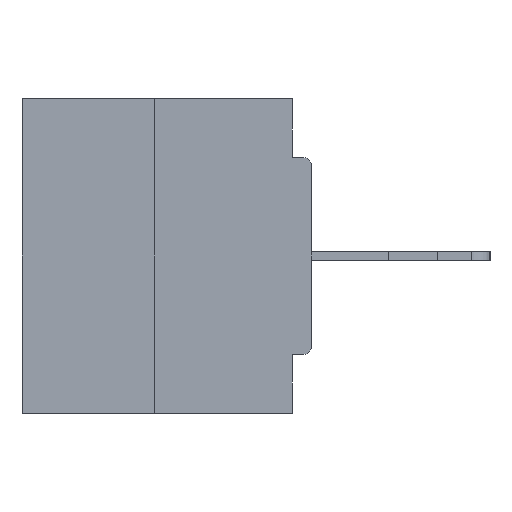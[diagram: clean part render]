
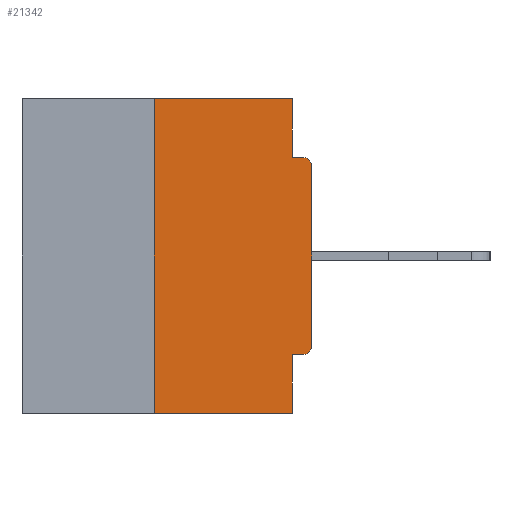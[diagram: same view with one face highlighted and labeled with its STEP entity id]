
A CAD part, left-side view. The second image highlights one B-rep face of the part: STEP entity #21342.
In plain terms, the highlighted planar face has unit normal (-1, 0, 0).
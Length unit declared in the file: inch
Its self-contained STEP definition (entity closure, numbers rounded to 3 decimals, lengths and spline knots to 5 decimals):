
#520 = DIRECTION ( 'NONE',  ( 1., 0., 0. ) ) ;
#844 = DIRECTION ( 'NONE',  ( 0., -1., 0. ) ) ;
#1271 = CARTESIAN_POINT ( 'NONE',  ( 0., 0.031, 0. ) ) ;
#1553 = VERTEX_POINT ( 'NONE', #24819 ) ;
#1582 = VERTEX_POINT ( 'NONE', #28336 ) ;
#1610 = VECTOR ( 'NONE', #22622, 39.37008 ) ;
#2001 = CIRCLE ( 'NONE', #3711, 0.015 ) ;
#2965 = VERTEX_POINT ( 'NONE', #4468 ) ;
#3505 = VECTOR ( 'NONE', #28901, 39.37008 ) ;
#3711 = AXIS2_PLACEMENT_3D ( 'NONE', #12974, #24083, #13518 ) ;
#3840 = VECTOR ( 'NONE', #9490, 39.37008 ) ;
#3979 = EDGE_CURVE ( 'NONE', #10822, #13764, #24867, .T. ) ;
#4160 = VECTOR ( 'NONE', #13693, 39.37008 ) ;
#4359 = CARTESIAN_POINT ( 'NONE',  ( 0., 0.015, -0.4065 ) ) ;
#4405 = DIRECTION ( 'NONE',  ( 0., 0., -1. ) ) ;
#4468 = CARTESIAN_POINT ( 'NONE',  ( 0., 0.25, -0.5 ) ) ;
#5059 = DIRECTION ( 'NONE',  ( 0., 0., 1. ) ) ;
#5913 = ORIENTED_EDGE ( 'NONE', *, *, #20773, .T. ) ;
#6026 = CARTESIAN_POINT ( 'NONE',  ( 0., 0., -0.3915 ) ) ;
#6584 = EDGE_LOOP ( 'NONE', ( #23778, #14687, #17450, #22697, #16497, #25538, #15675, #5913, #7654, #16845 ) ) ;
#7648 = EDGE_CURVE ( 'NONE', #10822, #25577, #26521, .T. ) ;
#7654 = ORIENTED_EDGE ( 'NONE', *, *, #25729, .F. ) ;
#8344 = CARTESIAN_POINT ( 'NONE',  ( 0., 0.031, -0.5 ) ) ;
#8827 = CARTESIAN_POINT ( 'NONE',  ( 0., 0., -0.0935 ) ) ;
#8965 = CARTESIAN_POINT ( 'NONE',  ( 0., 0.25, 0. ) ) ;
#9369 = DIRECTION ( 'NONE',  ( -1., 0., 0. ) ) ;
#9383 = VECTOR ( 'NONE', #10090, 39.37008 ) ;
#9490 = DIRECTION ( 'NONE',  ( 0., -1., 0. ) ) ;
#9552 = VERTEX_POINT ( 'NONE', #8965 ) ;
#9813 = CARTESIAN_POINT ( 'NONE',  ( 0., 0., 0. ) ) ;
#10090 = DIRECTION ( 'NONE',  ( 0., 1., 0. ) ) ;
#10709 = EDGE_CURVE ( 'NONE', #9552, #1582, #19611, .T. ) ;
#10822 = VERTEX_POINT ( 'NONE', #4359 ) ;
#11756 = VECTOR ( 'NONE', #5059, 39.37008 ) ;
#11995 = CARTESIAN_POINT ( 'NONE',  ( 0., 0.46, -0.5 ) ) ;
#12761 = CARTESIAN_POINT ( 'NONE',  ( 0., 0., -0.4065 ) ) ;
#12850 = LINE ( 'NONE', #32084, #11756 ) ;
#12974 = CARTESIAN_POINT ( 'NONE',  ( 0., 0.015, -0.1085 ) ) ;
#13419 = EDGE_CURVE ( 'NONE', #1582, #26879, #32898, .T. ) ;
#13518 = DIRECTION ( 'NONE',  ( 0., 0., -1. ) ) ;
#13693 = DIRECTION ( 'NONE',  ( 0., 0., -1. ) ) ;
#13764 = VERTEX_POINT ( 'NONE', #6026 ) ;
#14360 = CARTESIAN_POINT ( 'NONE',  ( 0., 0.015, -0.0935 ) ) ;
#14687 = ORIENTED_EDGE ( 'NONE', *, *, #23258, .F. ) ;
#15602 = AXIS2_PLACEMENT_3D ( 'NONE', #24758, #520, #33209 ) ;
#15675 = ORIENTED_EDGE ( 'NONE', *, *, #17492, .T. ) ;
#15985 = CARTESIAN_POINT ( 'NONE',  ( 0., 0.031, -0.5 ) ) ;
#16497 = ORIENTED_EDGE ( 'NONE', *, *, #7648, .F. ) ;
#16814 = PLANE ( 'NONE',  #15602 ) ;
#16845 = ORIENTED_EDGE ( 'NONE', *, *, #13419, .F. ) ;
#16994 = AXIS2_PLACEMENT_3D ( 'NONE', #33567, #9369, #4405 ) ;
#17450 = ORIENTED_EDGE ( 'NONE', *, *, #23168, .T. ) ;
#17492 = EDGE_CURVE ( 'NONE', #13764, #1553, #26252, .T. ) ;
#17572 = VECTOR ( 'NONE', #844, 39.37008 ) ;
#19362 = EDGE_CURVE ( 'NONE', #25577, #23999, #26908, .T. ) ;
#19474 = LINE ( 'NONE', #8827, #1610 ) ;
#19611 = LINE ( 'NONE', #27368, #17572 ) ;
#20773 = EDGE_CURVE ( 'NONE', #1553, #33858, #2001, .T. ) ;
#20934 = CARTESIAN_POINT ( 'NONE',  ( 0., 0.031, -0.0935 ) ) ;
#21342 = ADVANCED_FACE ( 'NONE', ( #30053 ), #16814, .F. ) ;
#22622 = DIRECTION ( 'NONE',  ( 0., -1., 0. ) ) ;
#22697 = ORIENTED_EDGE ( 'NONE', *, *, #19362, .F. ) ;
#23168 = EDGE_CURVE ( 'NONE', #2965, #23999, #25238, .T. ) ;
#23258 = EDGE_CURVE ( 'NONE', #2965, #9552, #12850, .T. ) ;
#23778 = ORIENTED_EDGE ( 'NONE', *, *, #10709, .F. ) ;
#23812 = VECTOR ( 'NONE', #27434, 39.37008 ) ;
#23999 = VERTEX_POINT ( 'NONE', #8344 ) ;
#24083 = DIRECTION ( 'NONE',  ( -1., 0., 0. ) ) ;
#24758 = CARTESIAN_POINT ( 'NONE',  ( 0., 0.46, 0. ) ) ;
#24819 = CARTESIAN_POINT ( 'NONE',  ( 0., 0., -0.1085 ) ) ;
#24867 = CIRCLE ( 'NONE', #16994, 0.015 ) ;
#25238 = LINE ( 'NONE', #11995, #3840 ) ;
#25538 = ORIENTED_EDGE ( 'NONE', *, *, #3979, .T. ) ;
#25577 = VERTEX_POINT ( 'NONE', #32673 ) ;
#25729 = EDGE_CURVE ( 'NONE', #26879, #33858, #19474, .T. ) ;
#26252 = LINE ( 'NONE', #9813, #3505 ) ;
#26521 = LINE ( 'NONE', #12761, #9383 ) ;
#26879 = VERTEX_POINT ( 'NONE', #20934 ) ;
#26908 = LINE ( 'NONE', #15985, #4160 ) ;
#27368 = CARTESIAN_POINT ( 'NONE',  ( 0., 0.46, 0. ) ) ;
#27434 = DIRECTION ( 'NONE',  ( 0., 0., -1. ) ) ;
#28336 = CARTESIAN_POINT ( 'NONE',  ( 0., 0.031, 0. ) ) ;
#28901 = DIRECTION ( 'NONE',  ( 0., 0., 1. ) ) ;
#30053 = FACE_OUTER_BOUND ( 'NONE', #6584, .T. ) ;
#32084 = CARTESIAN_POINT ( 'NONE',  ( 0., 0.25, 0. ) ) ;
#32673 = CARTESIAN_POINT ( 'NONE',  ( 0., 0.031, -0.4065 ) ) ;
#32898 = LINE ( 'NONE', #1271, #23812 ) ;
#33209 = DIRECTION ( 'NONE',  ( 0., 0., -1. ) ) ;
#33567 = CARTESIAN_POINT ( 'NONE',  ( 0., 0.015, -0.3915 ) ) ;
#33858 = VERTEX_POINT ( 'NONE', #14360 ) ;
